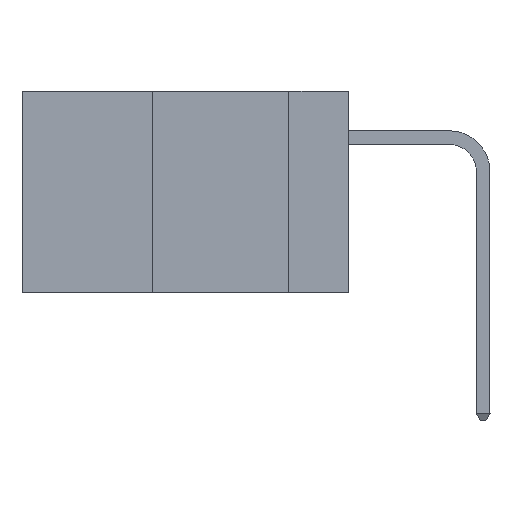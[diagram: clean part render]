
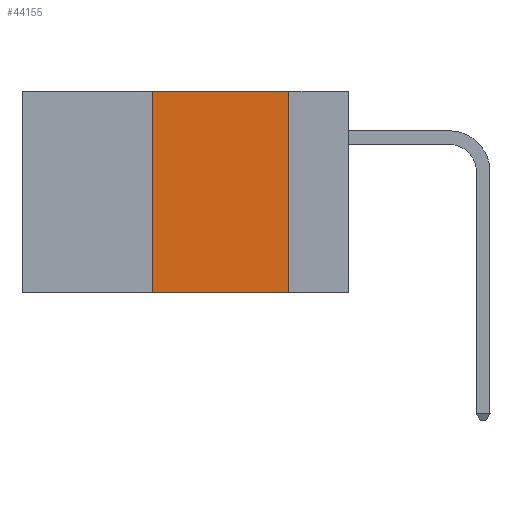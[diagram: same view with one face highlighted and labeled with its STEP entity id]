
A CAD part, left-side view. The second image highlights one B-rep face of the part: STEP entity #44155.
In plain terms, the highlighted planar face has unit normal (-1, 0, 0).
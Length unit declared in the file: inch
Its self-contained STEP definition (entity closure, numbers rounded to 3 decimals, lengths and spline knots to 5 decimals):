
#730 = LINE ( 'NONE', #43102, #39219 ) ;
#1482 = CARTESIAN_POINT ( 'NONE',  ( 0., 0.36, 0. ) ) ;
#3767 = DIRECTION ( 'NONE',  ( 0., 0., 1. ) ) ;
#5685 = VERTEX_POINT ( 'NONE', #39495 ) ;
#7460 = VECTOR ( 'NONE', #3767, 39.37008 ) ;
#7759 = CARTESIAN_POINT ( 'NONE',  ( 0., 0.36, 0. ) ) ;
#15776 = LINE ( 'NONE', #7759, #7460 ) ;
#19009 = LINE ( 'NONE', #41595, #42709 ) ;
#20049 = DIRECTION ( 'NONE',  ( 0., 0., -1. ) ) ;
#20667 = CARTESIAN_POINT ( 'NONE',  ( 0., 0.11, -0.37 ) ) ;
#21306 = CARTESIAN_POINT ( 'NONE',  ( 0., 0.6, -0.37 ) ) ;
#21354 = ORIENTED_EDGE ( 'NONE', *, *, #42655, .F. ) ;
#24649 = EDGE_CURVE ( 'NONE', #35638, #46612, #19009, .T. ) ;
#25732 = EDGE_LOOP ( 'NONE', ( #33962, #46983, #21354, #42120 ) ) ;
#25816 = LINE ( 'NONE', #21306, #45318 ) ;
#26311 = DIRECTION ( 'NONE',  ( 0., 0., -1. ) ) ;
#27658 = EDGE_CURVE ( 'NONE', #5685, #46612, #25816, .T. ) ;
#28592 = PLANE ( 'NONE',  #41862 ) ;
#29257 = VERTEX_POINT ( 'NONE', #1482 ) ;
#31310 = DIRECTION ( 'NONE',  ( 0., -1., 0. ) ) ;
#33962 = ORIENTED_EDGE ( 'NONE', *, *, #24649, .F. ) ;
#34222 = EDGE_CURVE ( 'NONE', #29257, #35638, #730, .T. ) ;
#35638 = VERTEX_POINT ( 'NONE', #40826 ) ;
#39219 = VECTOR ( 'NONE', #31310, 39.37008 ) ;
#39495 = CARTESIAN_POINT ( 'NONE',  ( 0., 0.36, -0.37 ) ) ;
#40108 = DIRECTION ( 'NONE',  ( 1., 0., 0. ) ) ;
#40826 = CARTESIAN_POINT ( 'NONE',  ( 0., 0.11, 0. ) ) ;
#41595 = CARTESIAN_POINT ( 'NONE',  ( 0., 0.11, 0. ) ) ;
#41862 = AXIS2_PLACEMENT_3D ( 'NONE', #46882, #40108, #20049 ) ;
#42120 = ORIENTED_EDGE ( 'NONE', *, *, #27658, .T. ) ;
#42655 = EDGE_CURVE ( 'NONE', #5685, #29257, #15776, .T. ) ;
#42709 = VECTOR ( 'NONE', #26311, 39.37008 ) ;
#43102 = CARTESIAN_POINT ( 'NONE',  ( 0., 0.6, 0. ) ) ;
#44155 = ADVANCED_FACE ( 'NONE', ( #46631 ), #28592, .F. ) ;
#45318 = VECTOR ( 'NONE', #49116, 39.37008 ) ;
#46612 = VERTEX_POINT ( 'NONE', #20667 ) ;
#46631 = FACE_OUTER_BOUND ( 'NONE', #25732, .T. ) ;
#46882 = CARTESIAN_POINT ( 'NONE',  ( 0., 0.6, 0. ) ) ;
#46983 = ORIENTED_EDGE ( 'NONE', *, *, #34222, .F. ) ;
#49116 = DIRECTION ( 'NONE',  ( 0., -1., 0. ) ) ;
